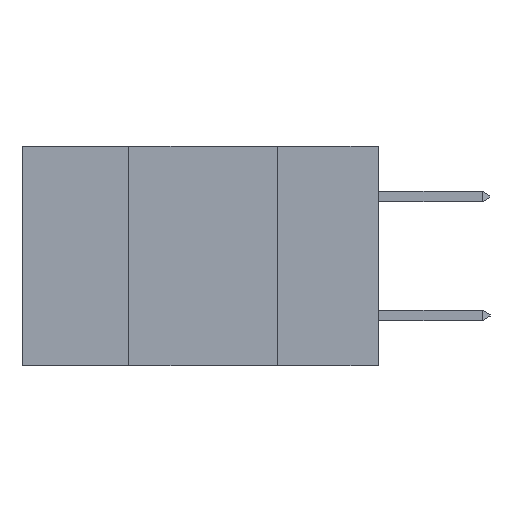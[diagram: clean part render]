
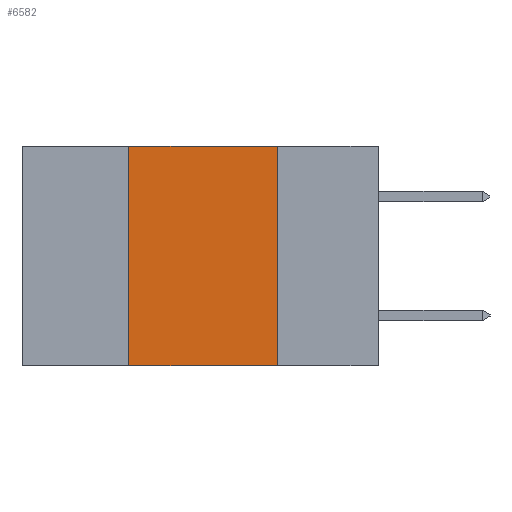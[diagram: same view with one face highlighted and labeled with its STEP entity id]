
A CAD part, left-side view. The second image highlights one B-rep face of the part: STEP entity #6582.
In plain terms, the highlighted planar face has unit normal (-1, 0, 0).
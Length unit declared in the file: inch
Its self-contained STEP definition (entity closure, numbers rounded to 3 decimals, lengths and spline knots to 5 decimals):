
#213 = DIRECTION ( 'NONE',  ( 0., -1., 0. ) ) ;
#269 = CARTESIAN_POINT ( 'NONE',  ( 0., 0.6, -0.37 ) ) ;
#958 = VERTEX_POINT ( 'NONE', #16001 ) ;
#1010 = VECTOR ( 'NONE', #2430, 39.37008 ) ;
#2430 = DIRECTION ( 'NONE',  ( 0., 0., -1. ) ) ;
#2799 = VERTEX_POINT ( 'NONE', #13551 ) ;
#3251 = CARTESIAN_POINT ( 'NONE',  ( 0., 0.42, -0.37 ) ) ;
#3261 = DIRECTION ( 'NONE',  ( 0., 0., 1. ) ) ;
#3422 = VECTOR ( 'NONE', #3261, 39.37008 ) ;
#4416 = EDGE_CURVE ( 'NONE', #958, #15195, #12630, .T. ) ;
#4680 = DIRECTION ( 'NONE',  ( 0., 0., -1. ) ) ;
#4704 = DIRECTION ( 'NONE',  ( 1., 0., 0. ) ) ;
#4715 = ORIENTED_EDGE ( 'NONE', *, *, #9627, .F. ) ;
#4740 = PLANE ( 'NONE',  #14806 ) ;
#5125 = LINE ( 'NONE', #14095, #1010 ) ;
#5256 = CARTESIAN_POINT ( 'NONE',  ( 0., 0.6, 0. ) ) ;
#5647 = ORIENTED_EDGE ( 'NONE', *, *, #4416, .T. ) ;
#5765 = VECTOR ( 'NONE', #7578, 39.37008 ) ;
#6582 = ADVANCED_FACE ( 'NONE', ( #13442 ), #4740, .F. ) ;
#6735 = EDGE_CURVE ( 'NONE', #958, #2799, #11180, .T. ) ;
#7578 = DIRECTION ( 'NONE',  ( 0., -1., 0. ) ) ;
#9045 = ORIENTED_EDGE ( 'NONE', *, *, #6735, .F. ) ;
#9598 = LINE ( 'NONE', #13324, #5765 ) ;
#9627 = EDGE_CURVE ( 'NONE', #2799, #12350, #9598, .T. ) ;
#11180 = LINE ( 'NONE', #3251, #3422 ) ;
#12350 = VERTEX_POINT ( 'NONE', #19063 ) ;
#12630 = LINE ( 'NONE', #269, #15974 ) ;
#13324 = CARTESIAN_POINT ( 'NONE',  ( 0., 0.6, 0. ) ) ;
#13442 = FACE_OUTER_BOUND ( 'NONE', #14754, .T. ) ;
#13551 = CARTESIAN_POINT ( 'NONE',  ( 0., 0.42, 0. ) ) ;
#14095 = CARTESIAN_POINT ( 'NONE',  ( 0., 0.17, -0.37 ) ) ;
#14754 = EDGE_LOOP ( 'NONE', ( #15338, #4715, #9045, #5647 ) ) ;
#14806 = AXIS2_PLACEMENT_3D ( 'NONE', #5256, #4704, #4680 ) ;
#15195 = VERTEX_POINT ( 'NONE', #18310 ) ;
#15338 = ORIENTED_EDGE ( 'NONE', *, *, #17337, .F. ) ;
#15974 = VECTOR ( 'NONE', #213, 39.37008 ) ;
#16001 = CARTESIAN_POINT ( 'NONE',  ( 0., 0.42, -0.37 ) ) ;
#17337 = EDGE_CURVE ( 'NONE', #12350, #15195, #5125, .T. ) ;
#18310 = CARTESIAN_POINT ( 'NONE',  ( 0., 0.17, -0.37 ) ) ;
#19063 = CARTESIAN_POINT ( 'NONE',  ( 0., 0.17, 0. ) ) ;
